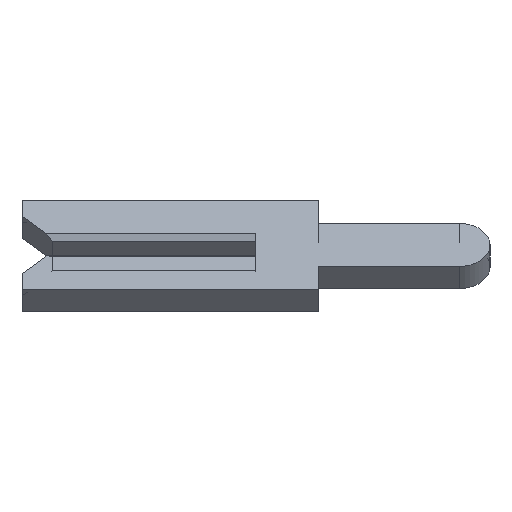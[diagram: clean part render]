
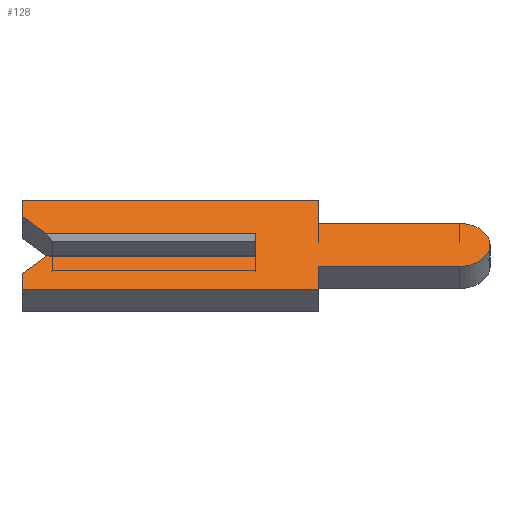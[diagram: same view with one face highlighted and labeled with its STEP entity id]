
A CAD part, left-side view. The second image highlights one B-rep face of the part: STEP entity #128.
In plain terms, the highlighted face is planar.
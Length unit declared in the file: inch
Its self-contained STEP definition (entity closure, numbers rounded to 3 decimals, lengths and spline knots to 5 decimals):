
#8 = DIRECTION ( 'NONE',  ( 0., 0.707, 0.707 ) ) ;
#18 = EDGE_CURVE ( 'NONE', #1076, #1737, #961, .T. ) ;
#30 = VECTOR ( 'NONE', #614, 39.37008 ) ;
#32 = VECTOR ( 'NONE', #1379, 39.37008 ) ;
#46 = CARTESIAN_POINT ( 'NONE',  ( -0.01, -0.04, -0.0195 ) ) ;
#58 = AXIS2_PLACEMENT_3D ( 'NONE', #798, #1277, #2767 ) ;
#90 = EDGE_CURVE ( 'NONE', #1737, #2064, #1886, .T. ) ;
#128 = ADVANCED_FACE ( 'NONE', ( #928 ), #1680, .F. ) ;
#162 = CARTESIAN_POINT ( 'NONE',  ( -0.01, -0.04, 0.0195 ) ) ;
#179 = EDGE_CURVE ( 'NONE', #2461, #2095, #594, .T. ) ;
#181 = LINE ( 'NONE', #567, #285 ) ;
#189 = ORIENTED_EDGE ( 'NONE', *, *, #18, .F. ) ;
#198 = EDGE_CURVE ( 'NONE', #1562, #2461, #1957, .T. ) ;
#240 = LINE ( 'NONE', #912, #1351 ) ;
#251 = CARTESIAN_POINT ( 'NONE',  ( -0.01, 0.1305, 0.0065 ) ) ;
#265 = CARTESIAN_POINT ( 'NONE',  ( -0.01, -0.04, -0.0195 ) ) ;
#281 = VECTOR ( 'NONE', #808, 39.37008 ) ;
#285 = VECTOR ( 'NONE', #488, 39.37008 ) ;
#288 = ORIENTED_EDGE ( 'NONE', *, *, #1415, .F. ) ;
#344 = VECTOR ( 'NONE', #8, 39.37008 ) ;
#353 = CARTESIAN_POINT ( 'NONE',  ( -0.01, -0.1305, -0.0195 ) ) ;
#466 = CARTESIAN_POINT ( 'NONE',  ( -0.01, 0.15, 0.026 ) ) ;
#488 = DIRECTION ( 'NONE',  ( 0., 0., 1. ) ) ;
#510 = EDGE_CURVE ( 'NONE', #1763, #666, #2355, .T. ) ;
#567 = CARTESIAN_POINT ( 'NONE',  ( -0.01, 0., 0.0065 ) ) ;
#577 = CARTESIAN_POINT ( 'NONE',  ( -0.01, -0.04, -0.04 ) ) ;
#594 = LINE ( 'NONE', #819, #1177 ) ;
#603 = ORIENTED_EDGE ( 'NONE', *, *, #2774, .F. ) ;
#614 = DIRECTION ( 'NONE',  ( 0., -1., 0. ) ) ;
#621 = VECTOR ( 'NONE', #1777, 39.37008 ) ;
#660 = EDGE_CURVE ( 'NONE', #1763, #905, #240, .T. ) ;
#666 = VERTEX_POINT ( 'NONE', #466 ) ;
#783 = CARTESIAN_POINT ( 'NONE',  ( -0.01, 0.15, -0.026 ) ) ;
#798 = CARTESIAN_POINT ( 'NONE',  ( -0.01, -0.1305, 0. ) ) ;
#801 = ORIENTED_EDGE ( 'NONE', *, *, #1995, .F. ) ;
#808 = DIRECTION ( 'NONE',  ( 0., -1., 0. ) ) ;
#819 = CARTESIAN_POINT ( 'NONE',  ( -0.01, 0.15, -0.026 ) ) ;
#824 = EDGE_CURVE ( 'NONE', #1622, #1076, #1207, .T. ) ;
#857 = DIRECTION ( 'NONE',  ( 0., -1., 0. ) ) ;
#876 = VERTEX_POINT ( 'NONE', #2658 ) ;
#905 = VERTEX_POINT ( 'NONE', #1991 ) ;
#912 = CARTESIAN_POINT ( 'NONE',  ( -0.01, 0.15, 0.01 ) ) ;
#914 = EDGE_CURVE ( 'NONE', #666, #1006, #955, .T. ) ;
#928 = FACE_OUTER_BOUND ( 'NONE', #1597, .T. ) ;
#955 = LINE ( 'NONE', #2364, #2481 ) ;
#961 = LINE ( 'NONE', #162, #281 ) ;
#990 = CARTESIAN_POINT ( 'NONE',  ( -0.01, -0.04, -0.04 ) ) ;
#1006 = VERTEX_POINT ( 'NONE', #1719 ) ;
#1054 = CARTESIAN_POINT ( 'NONE',  ( -0.01, -0.04, 0.04 ) ) ;
#1076 = VERTEX_POINT ( 'NONE', #1861 ) ;
#1083 = LINE ( 'NONE', #1750, #2146 ) ;
#1177 = VECTOR ( 'NONE', #2564, 39.37008 ) ;
#1207 = LINE ( 'NONE', #1054, #621 ) ;
#1218 = EDGE_CURVE ( 'NONE', #2064, #1399, #1329, .T. ) ;
#1262 = ORIENTED_EDGE ( 'NONE', *, *, #914, .F. ) ;
#1272 = CARTESIAN_POINT ( 'NONE',  ( -0.01, -0.04, 0.04 ) ) ;
#1274 = EDGE_CURVE ( 'NONE', #1399, #1562, #1822, .T. ) ;
#1277 = DIRECTION ( 'NONE',  ( 1., 0., 0. ) ) ;
#1329 = LINE ( 'NONE', #46, #32 ) ;
#1351 = VECTOR ( 'NONE', #857, 39.37008 ) ;
#1362 = ORIENTED_EDGE ( 'NONE', *, *, #824, .F. ) ;
#1379 = DIRECTION ( 'NONE',  ( 0., 1., 0. ) ) ;
#1399 = VERTEX_POINT ( 'NONE', #265 ) ;
#1415 = EDGE_CURVE ( 'NONE', #1501, #905, #181, .T. ) ;
#1431 = ORIENTED_EDGE ( 'NONE', *, *, #179, .F. ) ;
#1460 = VECTOR ( 'NONE', #1662, 39.37008 ) ;
#1480 = CARTESIAN_POINT ( 'NONE',  ( -0.01, -0.1305, 0. ) ) ;
#1501 = VERTEX_POINT ( 'NONE', #2018 ) ;
#1562 = VERTEX_POINT ( 'NONE', #577 ) ;
#1597 = EDGE_LOOP ( 'NONE', ( #2129, #288, #2778, #603, #1431, #2132, #1890, #2775, #2745, #189, #1362, #801, #1262, #1798 ) ) ;
#1622 = VERTEX_POINT ( 'NONE', #1272 ) ;
#1662 = DIRECTION ( 'NONE',  ( 0., 0., -1. ) ) ;
#1680 = PLANE ( 'NONE',  #2758 ) ;
#1687 = VECTOR ( 'NONE', #2748, 39.37008 ) ;
#1719 = CARTESIAN_POINT ( 'NONE',  ( -0.01, 0.15, 0.04 ) ) ;
#1737 = VERTEX_POINT ( 'NONE', #1915 ) ;
#1744 = DIRECTION ( 'NONE',  ( 0., -0.707, 0.707 ) ) ;
#1750 = CARTESIAN_POINT ( 'NONE',  ( -0.01, 0.1305, -0.0065 ) ) ;
#1757 = LINE ( 'NONE', #2318, #30 ) ;
#1763 = VERTEX_POINT ( 'NONE', #2108 ) ;
#1777 = DIRECTION ( 'NONE',  ( 0., 0., -1. ) ) ;
#1798 = ORIENTED_EDGE ( 'NONE', *, *, #510, .F. ) ;
#1822 = LINE ( 'NONE', #990, #1460 ) ;
#1861 = CARTESIAN_POINT ( 'NONE',  ( -0.01, -0.04, 0.0195 ) ) ;
#1886 = CIRCLE ( 'NONE', #58, 0.0195 ) ;
#1890 = ORIENTED_EDGE ( 'NONE', *, *, #1274, .F. ) ;
#1912 = DIRECTION ( 'NONE',  ( 0., 1., 0. ) ) ;
#1915 = CARTESIAN_POINT ( 'NONE',  ( -0.01, -0.1305, 0.0195 ) ) ;
#1927 = DIRECTION ( 'NONE',  ( 1., 0., 0. ) ) ;
#1957 = LINE ( 'NONE', #2522, #2257 ) ;
#1991 = CARTESIAN_POINT ( 'NONE',  ( -0.01, 0., 0.01 ) ) ;
#1995 = EDGE_CURVE ( 'NONE', #1006, #1622, #1757, .T. ) ;
#2018 = CARTESIAN_POINT ( 'NONE',  ( -0.01, 0., -0.01 ) ) ;
#2044 = EDGE_CURVE ( 'NONE', #876, #1501, #2255, .T. ) ;
#2064 = VERTEX_POINT ( 'NONE', #353 ) ;
#2095 = VERTEX_POINT ( 'NONE', #783 ) ;
#2108 = CARTESIAN_POINT ( 'NONE',  ( -0.01, 0.134, 0.01 ) ) ;
#2117 = DIRECTION ( 'NONE',  ( 0., 0., -1. ) ) ;
#2129 = ORIENTED_EDGE ( 'NONE', *, *, #660, .T. ) ;
#2132 = ORIENTED_EDGE ( 'NONE', *, *, #198, .F. ) ;
#2136 = CARTESIAN_POINT ( 'NONE',  ( -0.01, 0.15, -0.04 ) ) ;
#2146 = VECTOR ( 'NONE', #1744, 39.37008 ) ;
#2255 = LINE ( 'NONE', #2518, #1687 ) ;
#2257 = VECTOR ( 'NONE', #1912, 39.37008 ) ;
#2318 = CARTESIAN_POINT ( 'NONE',  ( -0.01, 0.15, 0.04 ) ) ;
#2355 = LINE ( 'NONE', #251, #344 ) ;
#2364 = CARTESIAN_POINT ( 'NONE',  ( -0.01, 0.15, 0.026 ) ) ;
#2461 = VERTEX_POINT ( 'NONE', #2136 ) ;
#2481 = VECTOR ( 'NONE', #2579, 39.37008 ) ;
#2518 = CARTESIAN_POINT ( 'NONE',  ( -0.01, -0.1305, -0.01 ) ) ;
#2522 = CARTESIAN_POINT ( 'NONE',  ( -0.01, 0.15, -0.04 ) ) ;
#2564 = DIRECTION ( 'NONE',  ( 0., 0., 1. ) ) ;
#2579 = DIRECTION ( 'NONE',  ( 0., 0., 1. ) ) ;
#2658 = CARTESIAN_POINT ( 'NONE',  ( -0.01, 0.134, -0.01 ) ) ;
#2745 = ORIENTED_EDGE ( 'NONE', *, *, #90, .F. ) ;
#2748 = DIRECTION ( 'NONE',  ( 0., -1., 0. ) ) ;
#2758 = AXIS2_PLACEMENT_3D ( 'NONE', #1480, #1927, #2117 ) ;
#2767 = DIRECTION ( 'NONE',  ( 0., 0., -1. ) ) ;
#2774 = EDGE_CURVE ( 'NONE', #2095, #876, #1083, .T. ) ;
#2775 = ORIENTED_EDGE ( 'NONE', *, *, #1218, .F. ) ;
#2778 = ORIENTED_EDGE ( 'NONE', *, *, #2044, .F. ) ;
